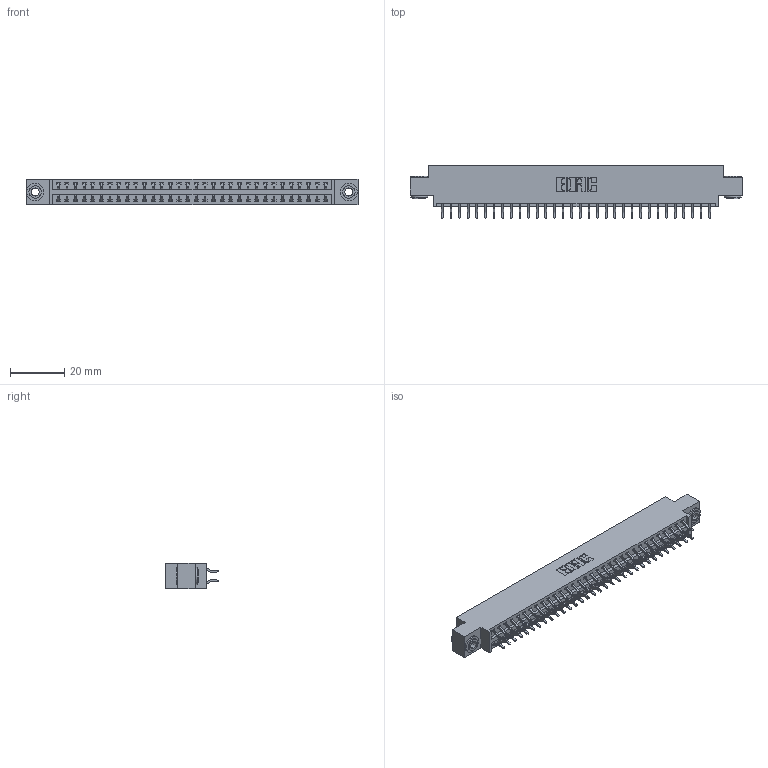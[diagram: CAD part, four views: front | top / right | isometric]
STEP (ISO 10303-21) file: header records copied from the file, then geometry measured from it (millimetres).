
FILE_DESCRIPTION (( 'STEP AP203' ), '1' );
FILE_NAME ('396-064-556-803.STEP', '2018-09-08T17:43:08', ( '' ), ( '' ), 'SwSTEP 2.0', 'SolidWorks 2016', '' );
FILE_SCHEMA (( 'CONFIG_CONTROL_DESIGN' ));
Length unit declared in the file: inch
Products named in the file (4): 346 Part_0.170 Offset - 0.156 Dia-TH; 345-292-001_556 Tail; 345-250-002_345-250-002-102; 396-064-556-803
Assembly tree (67 placements, depth 2):
  396-064-556-803
    346 Part_0.170 Offset - 0.156 Dia-TH
    345-292-001_556 Tail  x64
    345-250-002_345-250-002-102  x2
Bounding box: 122.17 x 19.57 x 9.4 mm (x, y, z)
Volume: 11698.1 mm3; surface area: 16256.9 mm2
Topology: 67 solids, 67 shells, 3876 faces, 11489 edges, 7570 vertices
Faces by surface type: plane 2586, cylinder 1282, cone 8
Entity records: 23232 total; most frequent: CARTESIAN_POINT 3835, ORIENTED_EDGE 3750, DIRECTION 3449, EDGE_CURVE 1875, VECTOR 1583, LINE 1583, VERTEX_POINT 1246, AXIS2_PLACEMENT_3D 933
